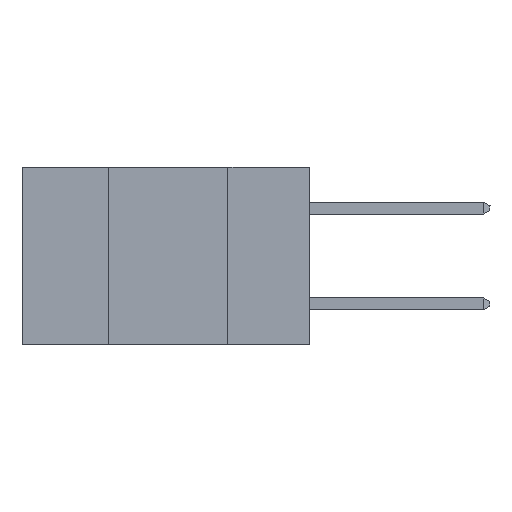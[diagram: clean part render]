
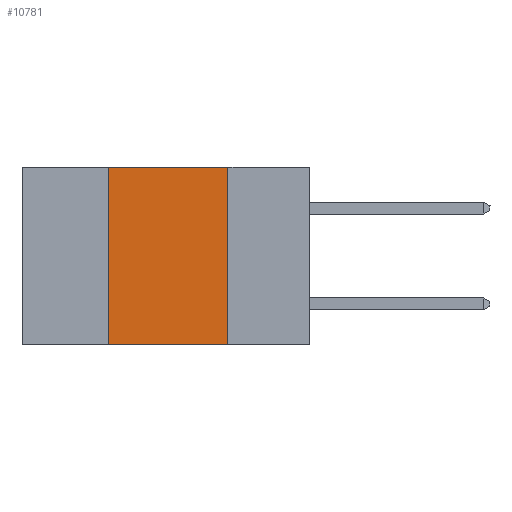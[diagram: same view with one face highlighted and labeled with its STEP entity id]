
A CAD part, left-side view. The second image highlights one B-rep face of the part: STEP entity #10781.
In plain terms, the highlighted planar face has unit normal (-1, 0, 0).
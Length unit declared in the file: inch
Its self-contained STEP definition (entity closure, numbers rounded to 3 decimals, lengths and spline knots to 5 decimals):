
#26 = CARTESIAN_POINT ( 'NONE',  ( 0., 0.6, -0.37 ) ) ;
#354 = LINE ( 'NONE', #3870, #8618 ) ;
#2441 = FACE_OUTER_BOUND ( 'NONE', #18377, .T. ) ;
#2702 = CARTESIAN_POINT ( 'NONE',  ( 0., 0.42, 0. ) ) ;
#3870 = CARTESIAN_POINT ( 'NONE',  ( 0., 0.42, 0. ) ) ;
#4492 = AXIS2_PLACEMENT_3D ( 'NONE', #13715, #6967, #18646 ) ;
#4757 = CARTESIAN_POINT ( 'NONE',  ( 0., 0.17, -0.37 ) ) ;
#4977 = CARTESIAN_POINT ( 'NONE',  ( 0., 0.17, 0. ) ) ;
#5166 = VECTOR ( 'NONE', #9969, 39.37008 ) ;
#5254 = DIRECTION ( 'NONE',  ( 0., -1., 0. ) ) ;
#5377 = ORIENTED_EDGE ( 'NONE', *, *, #8796, .F. ) ;
#6479 = VECTOR ( 'NONE', #15089, 39.37008 ) ;
#6702 = LINE ( 'NONE', #13671, #15102 ) ;
#6937 = ORIENTED_EDGE ( 'NONE', *, *, #18961, .F. ) ;
#6967 = DIRECTION ( 'NONE',  ( 1., 0., 0. ) ) ;
#7366 = VERTEX_POINT ( 'NONE', #4757 ) ;
#8618 = VECTOR ( 'NONE', #18888, 39.37008 ) ;
#8796 = EDGE_CURVE ( 'NONE', #20266, #7366, #21296, .T. ) ;
#9969 = DIRECTION ( 'NONE',  ( 0., -1., 0. ) ) ;
#10472 = ORIENTED_EDGE ( 'NONE', *, *, #14593, .F. ) ;
#10781 = ADVANCED_FACE ( 'NONE', ( #2441 ), #17010, .F. ) ;
#13671 = CARTESIAN_POINT ( 'NONE',  ( 0., 0.6, 0. ) ) ;
#13715 = CARTESIAN_POINT ( 'NONE',  ( 0., 0.6, 0. ) ) ;
#13751 = EDGE_CURVE ( 'NONE', #15748, #7366, #18487, .T. ) ;
#14593 = EDGE_CURVE ( 'NONE', #21117, #20266, #6702, .T. ) ;
#15089 = DIRECTION ( 'NONE',  ( 0., 0., -1. ) ) ;
#15102 = VECTOR ( 'NONE', #5254, 39.37008 ) ;
#15748 = VERTEX_POINT ( 'NONE', #20807 ) ;
#15808 = CARTESIAN_POINT ( 'NONE',  ( 0., 0.17, 0. ) ) ;
#17010 = PLANE ( 'NONE',  #4492 ) ;
#18377 = EDGE_LOOP ( 'NONE', ( #5377, #10472, #6937, #19435 ) ) ;
#18487 = LINE ( 'NONE', #26, #5166 ) ;
#18646 = DIRECTION ( 'NONE',  ( 0., 0., -1. ) ) ;
#18888 = DIRECTION ( 'NONE',  ( 0., 0., 1. ) ) ;
#18961 = EDGE_CURVE ( 'NONE', #15748, #21117, #354, .T. ) ;
#19435 = ORIENTED_EDGE ( 'NONE', *, *, #13751, .T. ) ;
#20266 = VERTEX_POINT ( 'NONE', #15808 ) ;
#20807 = CARTESIAN_POINT ( 'NONE',  ( 0., 0.42, -0.37 ) ) ;
#21117 = VERTEX_POINT ( 'NONE', #2702 ) ;
#21296 = LINE ( 'NONE', #4977, #6479 ) ;
